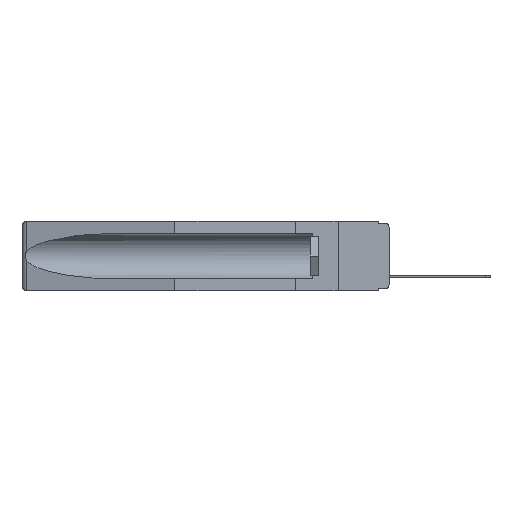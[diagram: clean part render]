
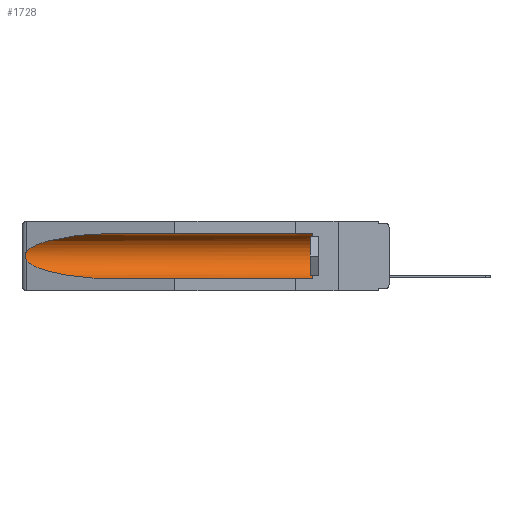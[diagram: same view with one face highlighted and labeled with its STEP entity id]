
A CAD part, left-side view. The second image highlights one B-rep face of the part: STEP entity #1728.
In plain terms, the highlighted cylindrical face has radius 2.857 mm (diameter 5.715 mm), a partial arc.
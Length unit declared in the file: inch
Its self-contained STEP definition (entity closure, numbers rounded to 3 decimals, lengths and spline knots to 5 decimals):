
#616 = ORIENTED_EDGE ( 'NONE', *, *, #15516, .T. ) ;
#755 = VECTOR ( 'NONE', #12380, 39.37008 ) ;
#756 = CARTESIAN_POINT ( 'NONE',  ( 0.21114, 1.30732, -0.284 ) ) ;
#940 = EDGE_CURVE ( 'NONE', #3884, #7442, #18351, .T. ) ;
#1728 = ADVANCED_FACE ( 'NONE', ( #16063 ), #12934, .F. ) ;
#2010 = DIRECTION ( 'NONE',  ( 0., 0., 1. ) ) ;
#2106 = CARTESIAN_POINT ( 'NONE',  ( 0.26655, 1.53094, -0.18657 ) ) ;
#2802 = VERTEX_POINT ( 'NONE', #3240 ) ;
#3240 = CARTESIAN_POINT ( 'NONE',  ( 0.155, 1.07973, -0.059 ) ) ;
#3328 = EDGE_LOOP ( 'NONE', ( #7466, #16802, #6056, #7281, #616, #14816 ) ) ;
#3884 = VERTEX_POINT ( 'NONE', #16457 ) ;
#5050 = CARTESIAN_POINT ( 'NONE',  ( 0.2673, 1.53269, -0.17917 ) ) ;
#5176 = CARTESIAN_POINT ( 'NONE',  ( 0.26537, 1.52718, -0.14972 ) ) ;
#5572 = CARTESIAN_POINT ( 'NONE',  ( 0.155, 1.07973, -0.284 ) ) ;
#5800 = EDGE_CURVE ( 'NONE', #2802, #8441, #16235, .T. ) ;
#5964 = CARTESIAN_POINT ( 'NONE',  ( 0.2675, 1.53308, -0.17534 ) ) ;
#6056 = ORIENTED_EDGE ( 'NONE', *, *, #940, .T. ) ;
#6151 = EDGE_CURVE ( 'NONE', #14224, #7442, #9357, .T. ) ;
#6459 = CARTESIAN_POINT ( 'NONE',  ( 0.21114, 1.30732, -0.059 ) ) ;
#7047 = EDGE_CURVE ( 'NONE', #8441, #3884, #17580, .T. ) ;
#7281 = ORIENTED_EDGE ( 'NONE', *, *, #6151, .F. ) ;
#7442 = VERTEX_POINT ( 'NONE', #9158 ) ;
#7466 = ORIENTED_EDGE ( 'NONE', *, *, #5800, .T. ) ;
#7570 = AXIS2_PLACEMENT_3D ( 'NONE', #13029, #17431, #9892 ) ;
#8081 = DIRECTION ( 'NONE',  ( 0., -1., 0. ) ) ;
#8084 = CARTESIAN_POINT ( 'NONE',  ( 0.26537, 1.52718, -0.19328 ) ) ;
#8441 = VERTEX_POINT ( 'NONE', #5176 ) ;
#8912 = CARTESIAN_POINT ( 'NONE',  ( 0.26597, 1.5296, -0.19026 ) ) ;
#9158 = CARTESIAN_POINT ( 'NONE',  ( 0.155, 1.07973, -0.284 ) ) ;
#9205 = CARTESIAN_POINT ( 'NONE',  ( 0.26654, 1.53092, -0.15636 ) ) ;
#9357 = LINE ( 'NONE', #9449, #755 ) ;
#9449 = CARTESIAN_POINT ( 'NONE',  ( 0.155, -0.30754, -0.284 ) ) ;
#9489 = CARTESIAN_POINT ( 'NONE',  ( 0.25451, 1.48313, -0.09465 ) ) ;
#9552 = CARTESIAN_POINT ( 'NONE',  ( 0.26537, 1.52718, -0.14972 ) ) ;
#9892 = DIRECTION ( 'NONE',  ( 0., 0., 1. ) ) ;
#10069 = CARTESIAN_POINT ( 'NONE',  ( 0.26537, 1.52718, -0.19328 ) ) ;
#11140 = CARTESIAN_POINT ( 'NONE',  ( 0.25451, 1.48313, -0.24835 ) ) ;
#12152 = CARTESIAN_POINT ( 'NONE',  ( 0.155, 0.126, -0.284 ) ) ;
#12380 = DIRECTION ( 'NONE',  ( 0., 1., 0. ) ) ;
#12435 = VECTOR ( 'NONE', #12915, 39.37008 ) ;
#12587 = CARTESIAN_POINT ( 'NONE',  ( 0.155, 0.126, -0.059 ) ) ;
#12915 = DIRECTION ( 'NONE',  ( 0., 1., 0. ) ) ;
#12934 = CYLINDRICAL_SURFACE ( 'NONE', #7570, 0.1125 ) ;
#13029 = CARTESIAN_POINT ( 'NONE',  ( 0.155, -0.30754, -0.1715 ) ) ;
#13693 = CARTESIAN_POINT ( 'NONE',  ( 0.155, 1.07973, -0.059 ) ) ;
#14224 = VERTEX_POINT ( 'NONE', #12152 ) ;
#14331 = CARTESIAN_POINT ( 'NONE',  ( 0.155, 0.126, -0.1715 ) ) ;
#14613 = EDGE_CURVE ( 'NONE', #19126, #2802, #17413, .T. ) ;
#14816 = ORIENTED_EDGE ( 'NONE', *, *, #14613, .T. ) ;
#15150 = CARTESIAN_POINT ( 'NONE',  ( 0.2673, 1.5327, -0.16383 ) ) ;
#15516 = EDGE_CURVE ( 'NONE', #14224, #19126, #19071, .T. ) ;
#15531 = CARTESIAN_POINT ( 'NONE',  ( 0.26537, 1.52718, -0.14972 ) ) ;
#15546 = CARTESIAN_POINT ( 'NONE',  ( 0.155, -0.30754, -0.059 ) ) ;
#16063 = FACE_OUTER_BOUND ( 'NONE', #3328, .T. ) ;
#16235 =( BOUNDED_CURVE ( )  B_SPLINE_CURVE ( 3, ( #13693, #6459, #9489, #15531 ),
 .UNSPECIFIED., .F., .F. ) 
 B_SPLINE_CURVE_WITH_KNOTS ( ( 4, 4 ),
 ( 4.71239, 6.08839 ),
 .UNSPECIFIED. ) 
 CURVE ( )  GEOMETRIC_REPRESENTATION_ITEM ( )  RATIONAL_B_SPLINE_CURVE ( ( 1., 0.848, 0.848, 1. ) ) 
 REPRESENTATION_ITEM ( '' )  );
#16457 = CARTESIAN_POINT ( 'NONE',  ( 0.26537, 1.52718, -0.19328 ) ) ;
#16802 = ORIENTED_EDGE ( 'NONE', *, *, #7047, .T. ) ;
#17413 = LINE ( 'NONE', #15546, #12435 ) ;
#17431 = DIRECTION ( 'NONE',  ( 0., 1., 0. ) ) ;
#17485 = AXIS2_PLACEMENT_3D ( 'NONE', #14331, #8081, #2010 ) ;
#17580 = B_SPLINE_CURVE_WITH_KNOTS ( 'NONE', 3,
 ( #9552, #18110, #9205, #15150, #18204, #5964, #5050, #2106, #8912, #8084 ),
 .UNSPECIFIED., .F., .F.,
 ( 4, 2, 2, 2, 4 ),
 ( 0., 0.00029, 0.00058, 0.00087, 0.00117 ),
 .UNSPECIFIED. ) ;
#18110 = CARTESIAN_POINT ( 'NONE',  ( 0.26597, 1.52961, -0.15275 ) ) ;
#18204 = CARTESIAN_POINT ( 'NONE',  ( 0.2675, 1.53308, -0.16763 ) ) ;
#18351 =( BOUNDED_CURVE ( )  B_SPLINE_CURVE ( 3, ( #10069, #11140, #756, #5572 ),
 .UNSPECIFIED., .F., .F. ) 
 B_SPLINE_CURVE_WITH_KNOTS ( ( 4, 4 ),
 ( 0.1948, 1.5708 ),
 .UNSPECIFIED. ) 
 CURVE ( )  GEOMETRIC_REPRESENTATION_ITEM ( )  RATIONAL_B_SPLINE_CURVE ( ( 1., 0.848, 0.848, 1. ) ) 
 REPRESENTATION_ITEM ( '' )  );
#19071 = CIRCLE ( 'NONE', #17485, 0.1125 ) ;
#19126 = VERTEX_POINT ( 'NONE', #12587 ) ;
